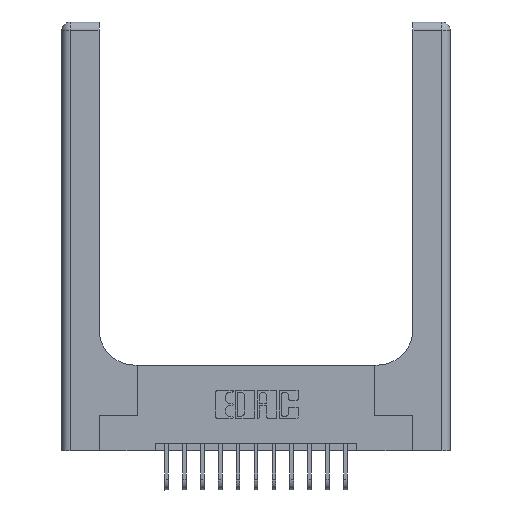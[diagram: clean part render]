
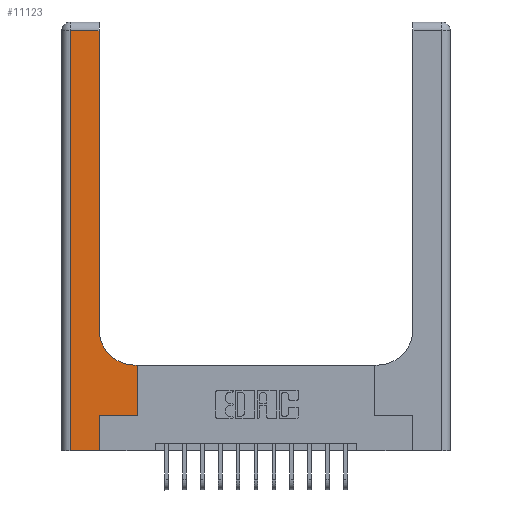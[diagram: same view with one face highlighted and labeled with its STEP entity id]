
A CAD part, top view. The second image highlights one B-rep face of the part: STEP entity #11123.
In plain terms, the highlighted planar face has unit normal (0, 0, 1).
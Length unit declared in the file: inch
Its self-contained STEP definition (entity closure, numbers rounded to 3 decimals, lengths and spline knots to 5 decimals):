
#94 = CARTESIAN_POINT ( 'NONE',  ( 0.06, 3., 0.37 ) ) ;
#214 = VERTEX_POINT ( 'NONE', #11455 ) ;
#431 = VECTOR ( 'NONE', #7267, 39.37008 ) ;
#439 = CARTESIAN_POINT ( 'NONE',  ( 0.26, 0.6, 0.37 ) ) ;
#701 = LINE ( 'NONE', #11629, #16450 ) ;
#814 = VECTOR ( 'NONE', #10579, 39.37008 ) ;
#837 = LINE ( 'NONE', #5603, #3267 ) ;
#875 = CARTESIAN_POINT ( 'NONE',  ( 0.06, 0., 0.37 ) ) ;
#1225 = VERTEX_POINT ( 'NONE', #6628 ) ;
#1343 = ORIENTED_EDGE ( 'NONE', *, *, #7773, .T. ) ;
#1539 = EDGE_CURVE ( 'NONE', #9840, #6785, #6629, .T. ) ;
#1684 = DIRECTION ( 'NONE',  ( 0., -1., 0. ) ) ;
#1961 = CARTESIAN_POINT ( 'NONE',  ( 0.26, 2.94, 0.37 ) ) ;
#2316 = DIRECTION ( 'NONE',  ( 0., 0., -1. ) ) ;
#2423 = VECTOR ( 'NONE', #15809, 39.37008 ) ;
#2577 = CARTESIAN_POINT ( 'NONE',  ( 0.265, 0.25, 0.37 ) ) ;
#3082 = EDGE_CURVE ( 'NONE', #6785, #12899, #12626, .T. ) ;
#3240 = VERTEX_POINT ( 'NONE', #5037 ) ;
#3267 = VECTOR ( 'NONE', #9918, 39.37008 ) ;
#3525 = VERTEX_POINT ( 'NONE', #14949 ) ;
#3988 = ORIENTED_EDGE ( 'NONE', *, *, #8436, .T. ) ;
#4176 = CARTESIAN_POINT ( 'NONE',  ( 0.26, 3., 0.37 ) ) ;
#4306 = CARTESIAN_POINT ( 'NONE',  ( 0., 0., 0.37 ) ) ;
#4612 = LINE ( 'NONE', #4176, #431 ) ;
#5037 = CARTESIAN_POINT ( 'NONE',  ( 0.26, 0.85, 0.37 ) ) ;
#5259 = VECTOR ( 'NONE', #10361, 39.37008 ) ;
#5603 = CARTESIAN_POINT ( 'NONE',  ( 0., 2.94, 0.37 ) ) ;
#6167 = LINE ( 'NONE', #439, #5259 ) ;
#6263 = ORIENTED_EDGE ( 'NONE', *, *, #8650, .T. ) ;
#6364 = ORIENTED_EDGE ( 'NONE', *, *, #1539, .T. ) ;
#6464 = DIRECTION ( 'NONE',  ( 0., 1., 0. ) ) ;
#6628 = CARTESIAN_POINT ( 'NONE',  ( 0.528, 0.6, 0.37 ) ) ;
#6629 = LINE ( 'NONE', #94, #17070 ) ;
#6648 = CARTESIAN_POINT ( 'NONE',  ( 0.06, 2.94, 0.37 ) ) ;
#6664 = DIRECTION ( 'NONE',  ( -1., 0., 0. ) ) ;
#6785 = VERTEX_POINT ( 'NONE', #875 ) ;
#7253 = FACE_OUTER_BOUND ( 'NONE', #14962, .T. ) ;
#7267 = DIRECTION ( 'NONE',  ( 0., 1., 0. ) ) ;
#7590 = EDGE_CURVE ( 'NONE', #3240, #15721, #4612, .T. ) ;
#7773 = EDGE_CURVE ( 'NONE', #3525, #3240, #11077, .T. ) ;
#7848 = VECTOR ( 'NONE', #6464, 39.37008 ) ;
#8117 = LINE ( 'NONE', #15022, #814 ) ;
#8436 = EDGE_CURVE ( 'NONE', #15721, #9840, #837, .T. ) ;
#8649 = CARTESIAN_POINT ( 'NONE',  ( 0.265, 0., 0.37 ) ) ;
#8650 = EDGE_CURVE ( 'NONE', #214, #1225, #8117, .T. ) ;
#8811 = ORIENTED_EDGE ( 'NONE', *, *, #14792, .T. ) ;
#9680 = EDGE_CURVE ( 'NONE', #12899, #10040, #13854, .T. ) ;
#9840 = VERTEX_POINT ( 'NONE', #6648 ) ;
#9918 = DIRECTION ( 'NONE',  ( -1., 0., 0. ) ) ;
#10040 = VERTEX_POINT ( 'NONE', #2577 ) ;
#10310 = DIRECTION ( 'NONE',  ( 1., 0., 0. ) ) ;
#10361 = DIRECTION ( 'NONE',  ( -1., 0., 0. ) ) ;
#10579 = DIRECTION ( 'NONE',  ( 0., 1., 0. ) ) ;
#10693 = CARTESIAN_POINT ( 'NONE',  ( 0.51, 0.85, 0.37 ) ) ;
#10967 = EDGE_CURVE ( 'NONE', #1225, #3525, #6167, .T. ) ;
#11077 = CIRCLE ( 'NONE', #14830, 0.25 ) ;
#11123 = ADVANCED_FACE ( 'NONE', ( #7253 ), #12260, .F. ) ;
#11319 = AXIS2_PLACEMENT_3D ( 'NONE', #14976, #13674, #6664 ) ;
#11330 = ORIENTED_EDGE ( 'NONE', *, *, #9680, .T. ) ;
#11455 = CARTESIAN_POINT ( 'NONE',  ( 0.528, 0.25, 0.37 ) ) ;
#11629 = CARTESIAN_POINT ( 'NONE',  ( 0.265, 0.25, 0.37 ) ) ;
#12240 = CARTESIAN_POINT ( 'NONE',  ( 0.265, 0., 0.37 ) ) ;
#12260 = PLANE ( 'NONE',  #11319 ) ;
#12626 = LINE ( 'NONE', #4306, #2423 ) ;
#12899 = VERTEX_POINT ( 'NONE', #12240 ) ;
#13107 = ORIENTED_EDGE ( 'NONE', *, *, #7590, .T. ) ;
#13674 = DIRECTION ( 'NONE',  ( 0., 0., -1. ) ) ;
#13698 = DIRECTION ( 'NONE',  ( 1., 0., 0. ) ) ;
#13854 = LINE ( 'NONE', #8649, #7848 ) ;
#14792 = EDGE_CURVE ( 'NONE', #10040, #214, #701, .T. ) ;
#14830 = AXIS2_PLACEMENT_3D ( 'NONE', #10693, #2316, #13698 ) ;
#14949 = CARTESIAN_POINT ( 'NONE',  ( 0.51, 0.6, 0.37 ) ) ;
#14962 = EDGE_LOOP ( 'NONE', ( #13107, #3988, #6364, #18065, #11330, #8811, #6263, #17267, #1343 ) ) ;
#14976 = CARTESIAN_POINT ( 'NONE',  ( 0., 3., 0.37 ) ) ;
#15022 = CARTESIAN_POINT ( 'NONE',  ( 0.528, 0.25, 0.37 ) ) ;
#15721 = VERTEX_POINT ( 'NONE', #1961 ) ;
#15809 = DIRECTION ( 'NONE',  ( 1., 0., 0. ) ) ;
#16450 = VECTOR ( 'NONE', #10310, 39.37008 ) ;
#17070 = VECTOR ( 'NONE', #1684, 39.37008 ) ;
#17267 = ORIENTED_EDGE ( 'NONE', *, *, #10967, .T. ) ;
#18065 = ORIENTED_EDGE ( 'NONE', *, *, #3082, .T. ) ;
